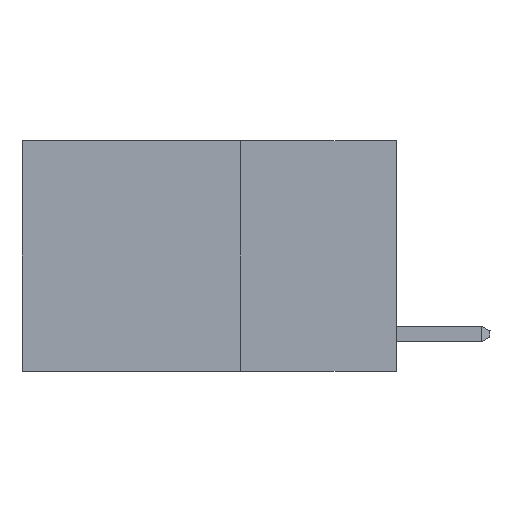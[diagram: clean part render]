
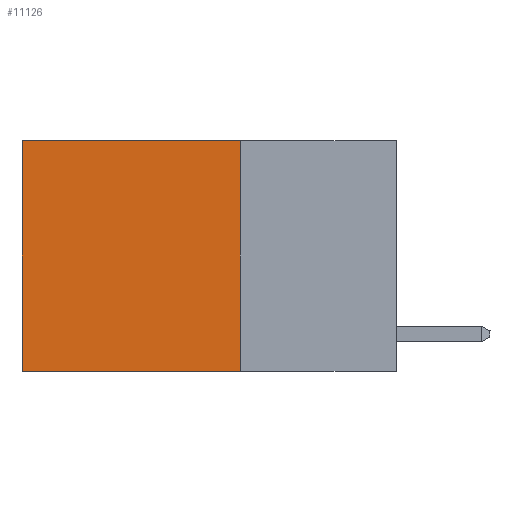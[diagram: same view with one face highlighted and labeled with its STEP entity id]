
A CAD part, left-side view. The second image highlights one B-rep face of the part: STEP entity #11126.
In plain terms, the highlighted planar face has unit normal (-1, 0, 0).
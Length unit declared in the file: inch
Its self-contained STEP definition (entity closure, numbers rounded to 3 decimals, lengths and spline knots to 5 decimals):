
#421 = DIRECTION ( 'NONE',  ( 0., 0., -1. ) ) ;
#1412 = EDGE_CURVE ( 'NONE', #3163, #12597, #13164, .T. ) ;
#1708 = CARTESIAN_POINT ( 'NONE',  ( 0.2625, 0.25, -0.37 ) ) ;
#1907 = VECTOR ( 'NONE', #10148, 39.37008 ) ;
#1913 = EDGE_CURVE ( 'NONE', #15761, #12597, #9258, .T. ) ;
#2787 = AXIS2_PLACEMENT_3D ( 'NONE', #15295, #7868, #421 ) ;
#3163 = VERTEX_POINT ( 'NONE', #13518 ) ;
#4416 = VECTOR ( 'NONE', #5990, 39.37008 ) ;
#4442 = DIRECTION ( 'NONE',  ( 0., 0., -1. ) ) ;
#4796 = CARTESIAN_POINT ( 'NONE',  ( 0.2625, 0.25, 0. ) ) ;
#4809 = DIRECTION ( 'NONE',  ( 0., 1., 0. ) ) ;
#4912 = LINE ( 'NONE', #7003, #10172 ) ;
#5300 = EDGE_LOOP ( 'NONE', ( #13794, #10056, #12143, #11265 ) ) ;
#5385 = CARTESIAN_POINT ( 'NONE',  ( 0.2625, 0.6, -0.37 ) ) ;
#5452 = PLANE ( 'NONE',  #2787 ) ;
#5766 = CARTESIAN_POINT ( 'NONE',  ( 0.2625, 0.25, 0. ) ) ;
#5990 = DIRECTION ( 'NONE',  ( 0., 1., 0. ) ) ;
#7003 = CARTESIAN_POINT ( 'NONE',  ( 0.2625, 0.25, 0. ) ) ;
#7868 = DIRECTION ( 'NONE',  ( 1., 0., 0. ) ) ;
#7910 = VECTOR ( 'NONE', #4809, 39.37008 ) ;
#8532 = CARTESIAN_POINT ( 'NONE',  ( 0.2625, 0.6, 0. ) ) ;
#9258 = LINE ( 'NONE', #14430, #7910 ) ;
#9407 = VERTEX_POINT ( 'NONE', #4796 ) ;
#10056 = ORIENTED_EDGE ( 'NONE', *, *, #1913, .F. ) ;
#10148 = DIRECTION ( 'NONE',  ( 0., 0., -1. ) ) ;
#10172 = VECTOR ( 'NONE', #4442, 39.37008 ) ;
#10295 = EDGE_CURVE ( 'NONE', #9407, #3163, #11041, .T. ) ;
#11041 = LINE ( 'NONE', #5766, #4416 ) ;
#11126 = ADVANCED_FACE ( 'NONE', ( #15283 ), #5452, .F. ) ;
#11265 = ORIENTED_EDGE ( 'NONE', *, *, #10295, .T. ) ;
#12143 = ORIENTED_EDGE ( 'NONE', *, *, #14432, .F. ) ;
#12597 = VERTEX_POINT ( 'NONE', #5385 ) ;
#13164 = LINE ( 'NONE', #8532, #1907 ) ;
#13518 = CARTESIAN_POINT ( 'NONE',  ( 0.2625, 0.6, 0. ) ) ;
#13794 = ORIENTED_EDGE ( 'NONE', *, *, #1412, .T. ) ;
#14430 = CARTESIAN_POINT ( 'NONE',  ( 0.2625, 0.25, -0.37 ) ) ;
#14432 = EDGE_CURVE ( 'NONE', #9407, #15761, #4912, .T. ) ;
#15283 = FACE_OUTER_BOUND ( 'NONE', #5300, .T. ) ;
#15295 = CARTESIAN_POINT ( 'NONE',  ( 0.2625, 0.25, 0. ) ) ;
#15761 = VERTEX_POINT ( 'NONE', #1708 ) ;
